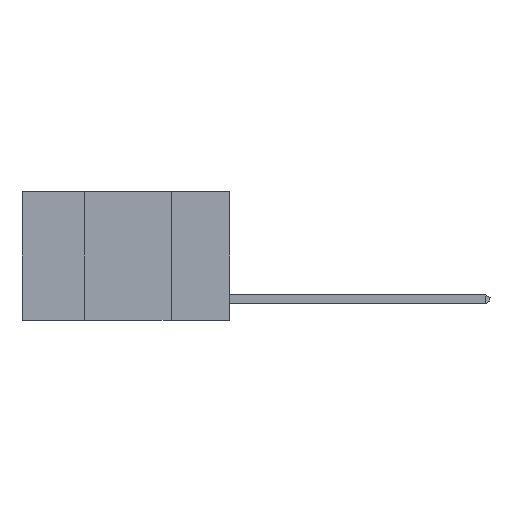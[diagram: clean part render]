
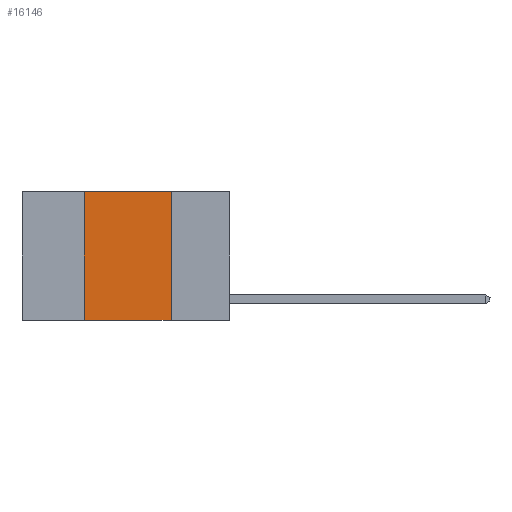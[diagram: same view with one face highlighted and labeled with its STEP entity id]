
A CAD part, left-side view. The second image highlights one B-rep face of the part: STEP entity #16146.
In plain terms, the highlighted planar face has unit normal (-1, 0, 0).
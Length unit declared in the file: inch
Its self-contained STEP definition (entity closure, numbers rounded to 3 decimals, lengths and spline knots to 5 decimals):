
#127 = CARTESIAN_POINT ( 'NONE',  ( 0., 0.42, 0. ) ) ;
#216 = EDGE_CURVE ( 'NONE', #5332, #19270, #17606, .T. ) ;
#1173 = EDGE_CURVE ( 'NONE', #5332, #13139, #14116, .T. ) ;
#2421 = EDGE_CURVE ( 'NONE', #25459, #13139, #4772, .T. ) ;
#3176 = VECTOR ( 'NONE', #3287, 39.37008 ) ;
#3287 = DIRECTION ( 'NONE',  ( 0., -1., 0. ) ) ;
#3360 = FACE_OUTER_BOUND ( 'NONE', #3473, .T. ) ;
#3473 = EDGE_LOOP ( 'NONE', ( #13416, #18797, #10657, #18164 ) ) ;
#4772 = LINE ( 'NONE', #6609, #7825 ) ;
#5332 = VERTEX_POINT ( 'NONE', #21433 ) ;
#5660 = CARTESIAN_POINT ( 'NONE',  ( 0., 0.17, 0. ) ) ;
#5765 = PLANE ( 'NONE',  #15186 ) ;
#6275 = VECTOR ( 'NONE', #22160, 39.37008 ) ;
#6473 = EDGE_CURVE ( 'NONE', #19270, #25459, #18495, .T. ) ;
#6609 = CARTESIAN_POINT ( 'NONE',  ( 0., 0.17, 0. ) ) ;
#6700 = CARTESIAN_POINT ( 'NONE',  ( 0., 0.42, 0. ) ) ;
#7825 = VECTOR ( 'NONE', #9163, 39.37008 ) ;
#9163 = DIRECTION ( 'NONE',  ( 0., 0., -1. ) ) ;
#10657 = ORIENTED_EDGE ( 'NONE', *, *, #216, .F. ) ;
#12042 = DIRECTION ( 'NONE',  ( 0., 0., -1. ) ) ;
#12319 = DIRECTION ( 'NONE',  ( 1., 0., 0. ) ) ;
#13139 = VERTEX_POINT ( 'NONE', #20611 ) ;
#13416 = ORIENTED_EDGE ( 'NONE', *, *, #2421, .F. ) ;
#14116 = LINE ( 'NONE', #22798, #3176 ) ;
#14465 = VECTOR ( 'NONE', #16215, 39.37008 ) ;
#15186 = AXIS2_PLACEMENT_3D ( 'NONE', #21011, #12319, #12042 ) ;
#16146 = ADVANCED_FACE ( 'NONE', ( #3360 ), #5765, .F. ) ;
#16215 = DIRECTION ( 'NONE',  ( 0., -1., 0. ) ) ;
#17606 = LINE ( 'NONE', #127, #6275 ) ;
#18164 = ORIENTED_EDGE ( 'NONE', *, *, #1173, .T. ) ;
#18495 = LINE ( 'NONE', #27039, #14465 ) ;
#18797 = ORIENTED_EDGE ( 'NONE', *, *, #6473, .F. ) ;
#19270 = VERTEX_POINT ( 'NONE', #6700 ) ;
#20611 = CARTESIAN_POINT ( 'NONE',  ( 0., 0.17, -0.37 ) ) ;
#21011 = CARTESIAN_POINT ( 'NONE',  ( 0., 0.6, 0. ) ) ;
#21433 = CARTESIAN_POINT ( 'NONE',  ( 0., 0.42, -0.37 ) ) ;
#22160 = DIRECTION ( 'NONE',  ( 0., 0., 1. ) ) ;
#22798 = CARTESIAN_POINT ( 'NONE',  ( 0., 0.6, -0.37 ) ) ;
#25459 = VERTEX_POINT ( 'NONE', #5660 ) ;
#27039 = CARTESIAN_POINT ( 'NONE',  ( 0., 0.6, 0. ) ) ;
